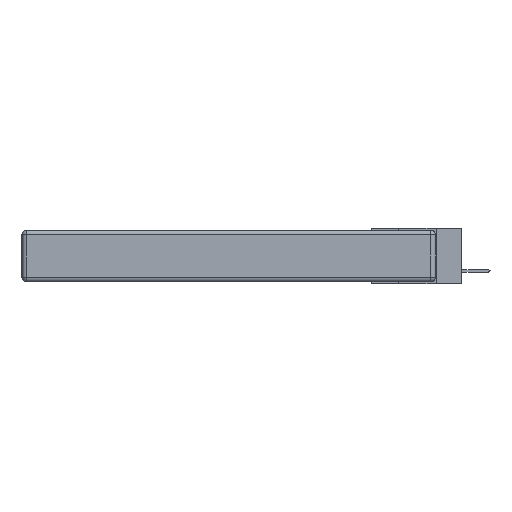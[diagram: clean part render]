
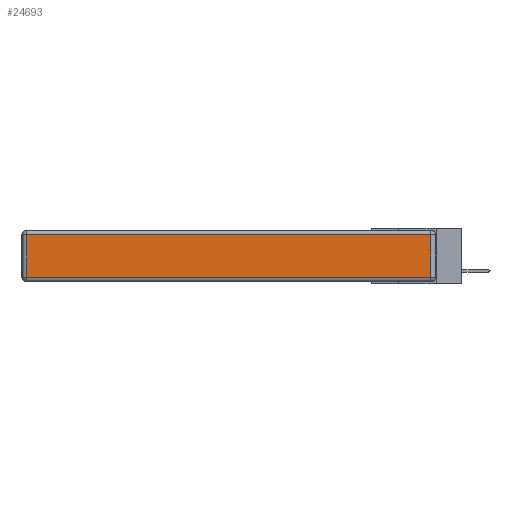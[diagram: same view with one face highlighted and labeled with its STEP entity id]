
A CAD part, left-side view. The second image highlights one B-rep face of the part: STEP entity #24693.
In plain terms, the highlighted planar face has unit normal (-1, 0, 0).
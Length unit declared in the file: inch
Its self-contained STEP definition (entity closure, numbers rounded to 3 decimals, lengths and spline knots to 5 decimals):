
#499 = CARTESIAN_POINT ( 'NONE',  ( 0., 0.03, -0.313 ) ) ;
#1877 = PLANE ( 'NONE',  #17108 ) ;
#2158 = ORIENTED_EDGE ( 'NONE', *, *, #16525, .T. ) ;
#2427 = VERTEX_POINT ( 'NONE', #9525 ) ;
#2550 = ORIENTED_EDGE ( 'NONE', *, *, #19970, .T. ) ;
#4293 = VECTOR ( 'NONE', #21767, 39.37008 ) ;
#4752 = VECTOR ( 'NONE', #12057, 39.37008 ) ;
#5805 = FACE_OUTER_BOUND ( 'NONE', #13223, .T. ) ;
#5812 = EDGE_CURVE ( 'NONE', #6606, #8900, #9714, .T. ) ;
#6606 = VERTEX_POINT ( 'NONE', #26134 ) ;
#7877 = VERTEX_POINT ( 'NONE', #13166 ) ;
#8900 = VERTEX_POINT ( 'NONE', #499 ) ;
#9525 = CARTESIAN_POINT ( 'NONE',  ( 0., 2.72, -0.03 ) ) ;
#9714 = LINE ( 'NONE', #12362, #21975 ) ;
#11730 = DIRECTION ( 'NONE',  ( 0., 1., 0. ) ) ;
#12057 = DIRECTION ( 'NONE',  ( 0., 0., 1. ) ) ;
#12362 = CARTESIAN_POINT ( 'NONE',  ( 0., 0., -0.313 ) ) ;
#12956 = VECTOR ( 'NONE', #11730, 39.37008 ) ;
#13151 = ORIENTED_EDGE ( 'NONE', *, *, #5812, .T. ) ;
#13166 = CARTESIAN_POINT ( 'NONE',  ( 0., 0.03, -0.03 ) ) ;
#13223 = EDGE_LOOP ( 'NONE', ( #13151, #20260, #2158, #2550 ) ) ;
#13546 = LINE ( 'NONE', #27077, #4752 ) ;
#16525 = EDGE_CURVE ( 'NONE', #7877, #2427, #26786, .T. ) ;
#17108 = AXIS2_PLACEMENT_3D ( 'NONE', #21303, #18829, #30813 ) ;
#18829 = DIRECTION ( 'NONE',  ( -1., 0., 0. ) ) ;
#19143 = EDGE_CURVE ( 'NONE', #8900, #7877, #13546, .T. ) ;
#19970 = EDGE_CURVE ( 'NONE', #2427, #6606, #28835, .T. ) ;
#20260 = ORIENTED_EDGE ( 'NONE', *, *, #19143, .T. ) ;
#21303 = CARTESIAN_POINT ( 'NONE',  ( 0., 0., -0.343 ) ) ;
#21364 = CARTESIAN_POINT ( 'NONE',  ( 0., 2.75, -0.03 ) ) ;
#21767 = DIRECTION ( 'NONE',  ( 0., 0., -1. ) ) ;
#21975 = VECTOR ( 'NONE', #29694, 39.37008 ) ;
#24693 = ADVANCED_FACE ( 'NONE', ( #5805 ), #1877, .T. ) ;
#26134 = CARTESIAN_POINT ( 'NONE',  ( 0., 2.72, -0.313 ) ) ;
#26786 = LINE ( 'NONE', #21364, #12956 ) ;
#27077 = CARTESIAN_POINT ( 'NONE',  ( 0., 0.03, -0.343 ) ) ;
#28835 = LINE ( 'NONE', #31710, #4293 ) ;
#29694 = DIRECTION ( 'NONE',  ( 0., -1., 0. ) ) ;
#30813 = DIRECTION ( 'NONE',  ( 0., 0., 1. ) ) ;
#31710 = CARTESIAN_POINT ( 'NONE',  ( 0., 2.72, -0.343 ) ) ;
